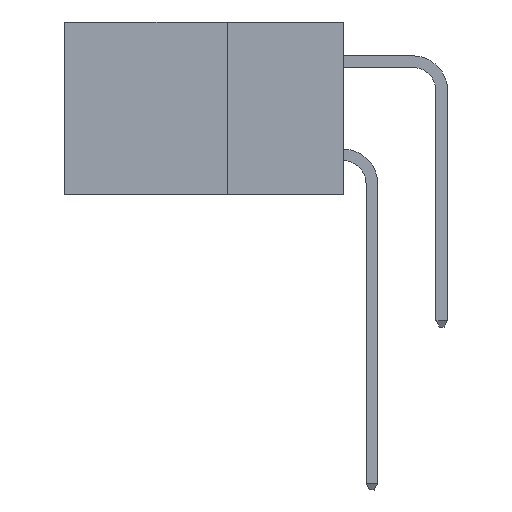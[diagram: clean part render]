
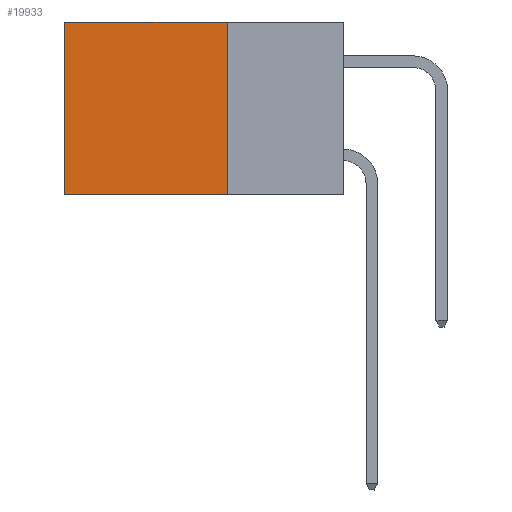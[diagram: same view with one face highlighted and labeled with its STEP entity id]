
A CAD part, left-side view. The second image highlights one B-rep face of the part: STEP entity #19933.
In plain terms, the highlighted planar face has unit normal (-1, 0, 0).
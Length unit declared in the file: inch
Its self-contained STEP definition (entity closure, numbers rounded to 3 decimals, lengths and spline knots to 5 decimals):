
#30 = ORIENTED_EDGE ( 'NONE', *, *, #12646, .F. ) ;
#396 = LINE ( 'NONE', #1797, #8657 ) ;
#458 = LINE ( 'NONE', #8135, #20684 ) ;
#1437 = VERTEX_POINT ( 'NONE', #7652 ) ;
#1797 = CARTESIAN_POINT ( 'NONE',  ( 0.298, 0.25, 0. ) ) ;
#2497 = VERTEX_POINT ( 'NONE', #7230 ) ;
#2687 = AXIS2_PLACEMENT_3D ( 'NONE', #16405, #17986, #8512 ) ;
#3415 = DIRECTION ( 'NONE',  ( 0., 0., -1. ) ) ;
#4298 = CARTESIAN_POINT ( 'NONE',  ( 0.298, 0.6, 0. ) ) ;
#5791 = VERTEX_POINT ( 'NONE', #19783 ) ;
#5801 = VECTOR ( 'NONE', #5920, 39.37008 ) ;
#5920 = DIRECTION ( 'NONE',  ( 0., 0., -1. ) ) ;
#5951 = EDGE_CURVE ( 'NONE', #20080, #2497, #18506, .T. ) ;
#6684 = EDGE_LOOP ( 'NONE', ( #7424, #17867, #30, #17173 ) ) ;
#7230 = CARTESIAN_POINT ( 'NONE',  ( 0.298, 0.6, -0.37 ) ) ;
#7424 = ORIENTED_EDGE ( 'NONE', *, *, #5951, .T. ) ;
#7652 = CARTESIAN_POINT ( 'NONE',  ( 0.298, 0.25, -0.37 ) ) ;
#8135 = CARTESIAN_POINT ( 'NONE',  ( 0.298, 0.25, 0. ) ) ;
#8512 = DIRECTION ( 'NONE',  ( 0., 0., -1. ) ) ;
#8657 = VECTOR ( 'NONE', #3415, 39.37008 ) ;
#10575 = EDGE_CURVE ( 'NONE', #5791, #20080, #458, .T. ) ;
#10615 = EDGE_CURVE ( 'NONE', #1437, #2497, #11966, .T. ) ;
#11966 = LINE ( 'NONE', #13044, #19763 ) ;
#12646 = EDGE_CURVE ( 'NONE', #5791, #1437, #396, .T. ) ;
#13044 = CARTESIAN_POINT ( 'NONE',  ( 0.298, 0.25, -0.37 ) ) ;
#13687 = CARTESIAN_POINT ( 'NONE',  ( 0.298, 0.6, 0. ) ) ;
#14197 = FACE_OUTER_BOUND ( 'NONE', #6684, .T. ) ;
#14619 = DIRECTION ( 'NONE',  ( 0., 1., 0. ) ) ;
#14858 = PLANE ( 'NONE',  #2687 ) ;
#16405 = CARTESIAN_POINT ( 'NONE',  ( 0.298, 0.25, 0. ) ) ;
#17173 = ORIENTED_EDGE ( 'NONE', *, *, #10575, .T. ) ;
#17867 = ORIENTED_EDGE ( 'NONE', *, *, #10615, .F. ) ;
#17986 = DIRECTION ( 'NONE',  ( 1., 0., 0. ) ) ;
#18506 = LINE ( 'NONE', #4298, #5801 ) ;
#19166 = DIRECTION ( 'NONE',  ( 0., 1., 0. ) ) ;
#19763 = VECTOR ( 'NONE', #14619, 39.37008 ) ;
#19783 = CARTESIAN_POINT ( 'NONE',  ( 0.298, 0.25, 0. ) ) ;
#19933 = ADVANCED_FACE ( 'NONE', ( #14197 ), #14858, .F. ) ;
#20080 = VERTEX_POINT ( 'NONE', #13687 ) ;
#20684 = VECTOR ( 'NONE', #19166, 39.37008 ) ;
